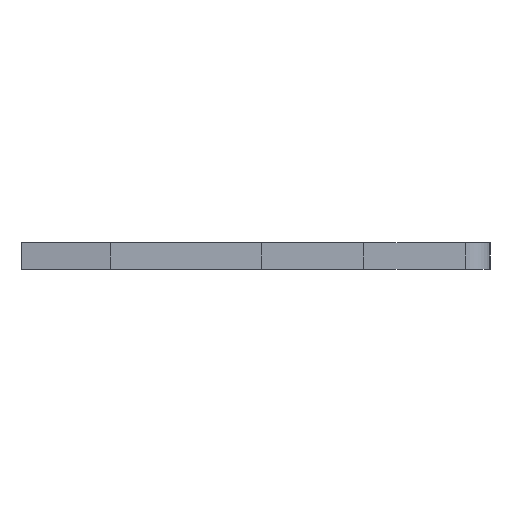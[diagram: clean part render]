
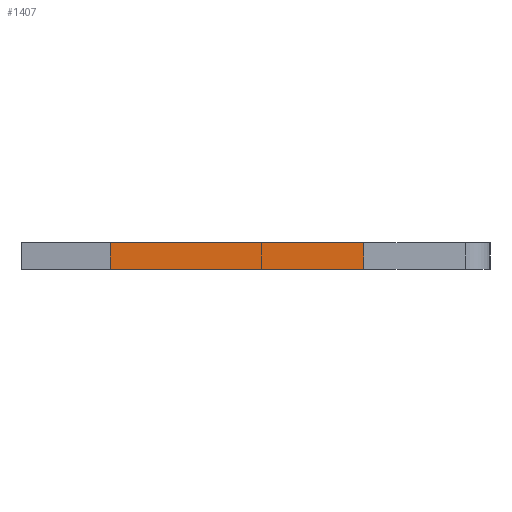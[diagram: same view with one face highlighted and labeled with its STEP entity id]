
A CAD part, left-side view. The second image highlights one B-rep face of the part: STEP entity #1407.
In plain terms, the highlighted face is planar.
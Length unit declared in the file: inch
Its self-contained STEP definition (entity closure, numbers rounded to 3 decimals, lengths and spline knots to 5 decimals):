
#7 = VERTEX_POINT ( 'NONE', #1574 ) ;
#18 = DIRECTION ( 'NONE',  ( -1., 0., 0. ) ) ;
#128 = VECTOR ( 'NONE', #1209, 39.37008 ) ;
#131 = EDGE_LOOP ( 'NONE', ( #918, #619, #2187, #1415 ) ) ;
#191 = AXIS2_PLACEMENT_3D ( 'NONE', #2153, #1827, #581 ) ;
#318 = VECTOR ( 'NONE', #463, 39.37008 ) ;
#331 = CARTESIAN_POINT ( 'NONE',  ( 0.013, -0.099, -0.0575 ) ) ;
#341 = VECTOR ( 'NONE', #1106, 39.37008 ) ;
#463 = DIRECTION ( 'NONE',  ( 0., 1., 0. ) ) ;
#581 = DIRECTION ( 'NONE',  ( 1., 0., 0. ) ) ;
#597 = VERTEX_POINT ( 'NONE', #656 ) ;
#619 = ORIENTED_EDGE ( 'NONE', *, *, #1152, .F. ) ;
#656 = CARTESIAN_POINT ( 'NONE',  ( -0.013, -0.099, -0.0575 ) ) ;
#731 = EDGE_CURVE ( 'NONE', #801, #7, #2016, .T. ) ;
#801 = VERTEX_POINT ( 'NONE', #331 ) ;
#828 = FACE_OUTER_BOUND ( 'NONE', #131, .T. ) ;
#880 = CARTESIAN_POINT ( 'NONE',  ( -0.013, 0.146, -0.0575 ) ) ;
#918 = ORIENTED_EDGE ( 'NONE', *, *, #1769, .T. ) ;
#1078 = LINE ( 'NONE', #1150, #318 ) ;
#1106 = DIRECTION ( 'NONE',  ( -1., 0., 0. ) ) ;
#1150 = CARTESIAN_POINT ( 'NONE',  ( -0.013, 0.146, -0.0575 ) ) ;
#1152 = EDGE_CURVE ( 'NONE', #7, #2099, #1192, .T. ) ;
#1179 = EDGE_CURVE ( 'NONE', #801, #597, #1753, .T. ) ;
#1192 = LINE ( 'NONE', #1778, #1382 ) ;
#1209 = DIRECTION ( 'NONE',  ( 0., 1., 0. ) ) ;
#1232 = CARTESIAN_POINT ( 'NONE',  ( 0.013, -0.099, -0.0575 ) ) ;
#1382 = VECTOR ( 'NONE', #18, 39.37008 ) ;
#1392 = CARTESIAN_POINT ( 'NONE',  ( 0.013, 0.146, -0.0575 ) ) ;
#1407 = ADVANCED_FACE ( 'NONE', ( #828 ), #1980, .F. ) ;
#1415 = ORIENTED_EDGE ( 'NONE', *, *, #1179, .T. ) ;
#1574 = CARTESIAN_POINT ( 'NONE',  ( 0.013, 0.146, -0.0575 ) ) ;
#1753 = LINE ( 'NONE', #1232, #341 ) ;
#1769 = EDGE_CURVE ( 'NONE', #597, #2099, #1078, .T. ) ;
#1778 = CARTESIAN_POINT ( 'NONE',  ( 0.013, 0.146, -0.0575 ) ) ;
#1827 = DIRECTION ( 'NONE',  ( 0., 0., 1. ) ) ;
#1980 = PLANE ( 'NONE',  #191 ) ;
#2016 = LINE ( 'NONE', #1392, #128 ) ;
#2099 = VERTEX_POINT ( 'NONE', #880 ) ;
#2153 = CARTESIAN_POINT ( 'NONE',  ( 0.013, 0.146, -0.0575 ) ) ;
#2187 = ORIENTED_EDGE ( 'NONE', *, *, #731, .F. ) ;
